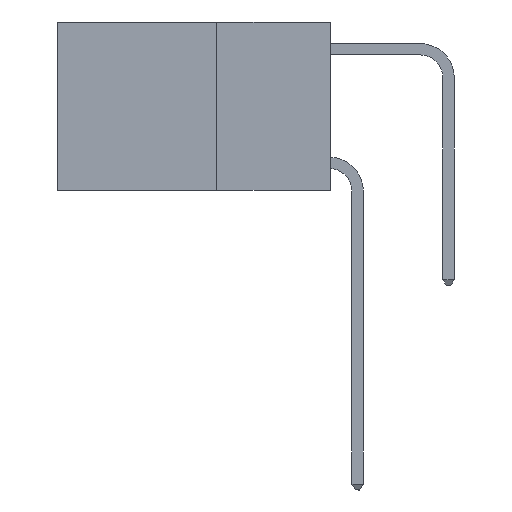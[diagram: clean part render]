
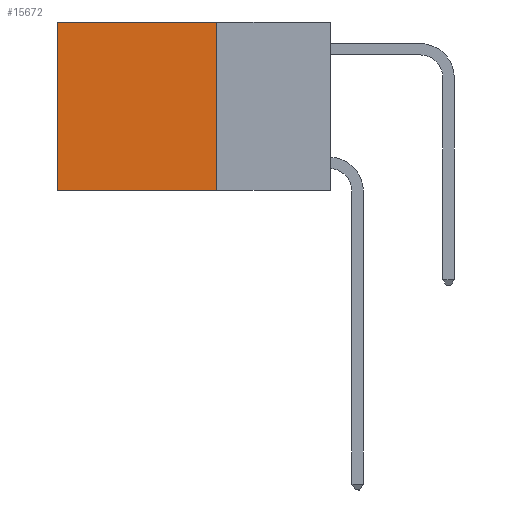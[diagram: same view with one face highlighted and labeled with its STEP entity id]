
A CAD part, left-side view. The second image highlights one B-rep face of the part: STEP entity #15672.
In plain terms, the highlighted planar face has unit normal (-1, 0, 0).
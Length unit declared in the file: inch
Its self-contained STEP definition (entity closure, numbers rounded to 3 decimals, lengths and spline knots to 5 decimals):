
#251 = ORIENTED_EDGE ( 'NONE', *, *, #10559, .F. ) ;
#400 = EDGE_CURVE ( 'NONE', #20774, #20108, #28490, .T. ) ;
#1124 = CARTESIAN_POINT ( 'NONE',  ( 0.2625, 0.25, 0. ) ) ;
#1740 = VERTEX_POINT ( 'NONE', #5349 ) ;
#4991 = DIRECTION ( 'NONE',  ( 0., 0., -1. ) ) ;
#5349 = CARTESIAN_POINT ( 'NONE',  ( 0.2625, 0.25, 0. ) ) ;
#5806 = ORIENTED_EDGE ( 'NONE', *, *, #18311, .T. ) ;
#6641 = DIRECTION ( 'NONE',  ( 1., 0., 0. ) ) ;
#7719 = CARTESIAN_POINT ( 'NONE',  ( 0.2625, 0.6, -0.37 ) ) ;
#9287 = VECTOR ( 'NONE', #29500, 39.37008 ) ;
#10120 = VERTEX_POINT ( 'NONE', #26364 ) ;
#10559 = EDGE_CURVE ( 'NONE', #10120, #20108, #34009, .T. ) ;
#15317 = EDGE_LOOP ( 'NONE', ( #18078, #251, #22436, #5806 ) ) ;
#15672 = ADVANCED_FACE ( 'NONE', ( #27526 ), #22348, .F. ) ;
#15925 = CARTESIAN_POINT ( 'NONE',  ( 0.2625, 0.25, -0.37 ) ) ;
#17347 = DIRECTION ( 'NONE',  ( 0., 0., -1. ) ) ;
#17947 = LINE ( 'NONE', #20712, #21423 ) ;
#18078 = ORIENTED_EDGE ( 'NONE', *, *, #400, .T. ) ;
#18210 = CARTESIAN_POINT ( 'NONE',  ( 0.2625, 0.6, 0. ) ) ;
#18311 = EDGE_CURVE ( 'NONE', #1740, #20774, #17947, .T. ) ;
#18538 = EDGE_CURVE ( 'NONE', #1740, #10120, #23804, .T. ) ;
#18692 = DIRECTION ( 'NONE',  ( 0., 1., 0. ) ) ;
#18961 = VECTOR ( 'NONE', #4991, 39.37008 ) ;
#19989 = AXIS2_PLACEMENT_3D ( 'NONE', #1124, #6641, #17347 ) ;
#20108 = VERTEX_POINT ( 'NONE', #7719 ) ;
#20712 = CARTESIAN_POINT ( 'NONE',  ( 0.2625, 0.25, 0. ) ) ;
#20774 = VERTEX_POINT ( 'NONE', #18210 ) ;
#21423 = VECTOR ( 'NONE', #30707, 39.37008 ) ;
#21548 = CARTESIAN_POINT ( 'NONE',  ( 0.2625, 0.25, 0. ) ) ;
#22348 = PLANE ( 'NONE',  #19989 ) ;
#22436 = ORIENTED_EDGE ( 'NONE', *, *, #18538, .F. ) ;
#23804 = LINE ( 'NONE', #21548, #9287 ) ;
#26364 = CARTESIAN_POINT ( 'NONE',  ( 0.2625, 0.25, -0.37 ) ) ;
#27073 = VECTOR ( 'NONE', #18692, 39.37008 ) ;
#27526 = FACE_OUTER_BOUND ( 'NONE', #15317, .T. ) ;
#28490 = LINE ( 'NONE', #31216, #18961 ) ;
#29500 = DIRECTION ( 'NONE',  ( 0., 0., -1. ) ) ;
#30707 = DIRECTION ( 'NONE',  ( 0., 1., 0. ) ) ;
#31216 = CARTESIAN_POINT ( 'NONE',  ( 0.2625, 0.6, 0. ) ) ;
#34009 = LINE ( 'NONE', #15925, #27073 ) ;
